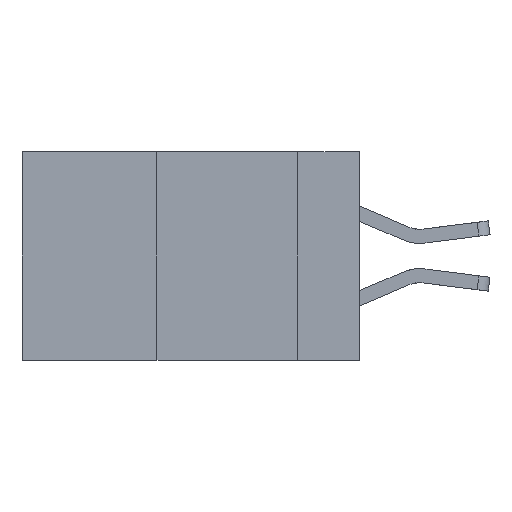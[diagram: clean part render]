
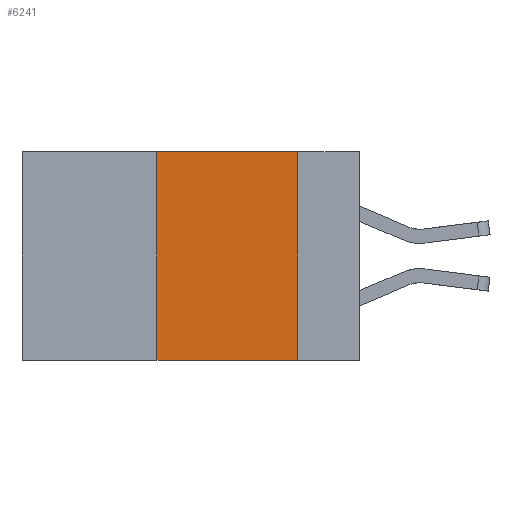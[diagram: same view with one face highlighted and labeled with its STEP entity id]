
A CAD part, left-side view. The second image highlights one B-rep face of the part: STEP entity #6241.
In plain terms, the highlighted planar face has unit normal (-1, 0, 0).
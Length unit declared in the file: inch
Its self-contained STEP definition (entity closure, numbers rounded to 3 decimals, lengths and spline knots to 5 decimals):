
#171 = EDGE_CURVE ( 'NONE', #8309, #9256, #8153, .T. ) ;
#611 = DIRECTION ( 'NONE',  ( 0., -1., 0. ) ) ;
#915 = VECTOR ( 'NONE', #8503, 39.37008 ) ;
#990 = CARTESIAN_POINT ( 'NONE',  ( 0., 0.11, 0. ) ) ;
#1024 = CARTESIAN_POINT ( 'NONE',  ( 0., 0.36, 0. ) ) ;
#1063 = EDGE_CURVE ( 'NONE', #8093, #8309, #2537, .T. ) ;
#1497 = CARTESIAN_POINT ( 'NONE',  ( 0., 0.6, -0.37 ) ) ;
#1522 = VERTEX_POINT ( 'NONE', #6733 ) ;
#1593 = CARTESIAN_POINT ( 'NONE',  ( 0., 0.36, -0.37 ) ) ;
#2333 = DIRECTION ( 'NONE',  ( 0., 0., -1. ) ) ;
#2420 = EDGE_CURVE ( 'NONE', #9256, #1522, #11046, .T. ) ;
#2537 = LINE ( 'NONE', #8388, #915 ) ;
#3002 = AXIS2_PLACEMENT_3D ( 'NONE', #4007, #9235, #7490 ) ;
#3263 = FACE_OUTER_BOUND ( 'NONE', #5438, .T. ) ;
#3592 = VECTOR ( 'NONE', #611, 39.37008 ) ;
#3877 = CARTESIAN_POINT ( 'NONE',  ( 0., 0.6, 0. ) ) ;
#4007 = CARTESIAN_POINT ( 'NONE',  ( 0., 0.6, 0. ) ) ;
#4191 = LINE ( 'NONE', #1497, #3592 ) ;
#4594 = ORIENTED_EDGE ( 'NONE', *, *, #5409, .T. ) ;
#4831 = VECTOR ( 'NONE', #4933, 39.37008 ) ;
#4891 = PLANE ( 'NONE',  #3002 ) ;
#4933 = DIRECTION ( 'NONE',  ( 0., -1., 0. ) ) ;
#5409 = EDGE_CURVE ( 'NONE', #8093, #1522, #4191, .T. ) ;
#5438 = EDGE_LOOP ( 'NONE', ( #10424, #8762, #6702, #4594 ) ) ;
#6241 = ADVANCED_FACE ( 'NONE', ( #3263 ), #4891, .F. ) ;
#6702 = ORIENTED_EDGE ( 'NONE', *, *, #1063, .F. ) ;
#6733 = CARTESIAN_POINT ( 'NONE',  ( 0., 0.11, -0.37 ) ) ;
#7490 = DIRECTION ( 'NONE',  ( 0., 0., -1. ) ) ;
#7570 = CARTESIAN_POINT ( 'NONE',  ( 0., 0.11, 0. ) ) ;
#8093 = VERTEX_POINT ( 'NONE', #1593 ) ;
#8153 = LINE ( 'NONE', #3877, #4831 ) ;
#8309 = VERTEX_POINT ( 'NONE', #1024 ) ;
#8388 = CARTESIAN_POINT ( 'NONE',  ( 0., 0.36, 0. ) ) ;
#8503 = DIRECTION ( 'NONE',  ( 0., 0., 1. ) ) ;
#8762 = ORIENTED_EDGE ( 'NONE', *, *, #171, .F. ) ;
#9235 = DIRECTION ( 'NONE',  ( 1., 0., 0. ) ) ;
#9256 = VERTEX_POINT ( 'NONE', #990 ) ;
#10128 = VECTOR ( 'NONE', #2333, 39.37008 ) ;
#10424 = ORIENTED_EDGE ( 'NONE', *, *, #2420, .F. ) ;
#11046 = LINE ( 'NONE', #7570, #10128 ) ;
